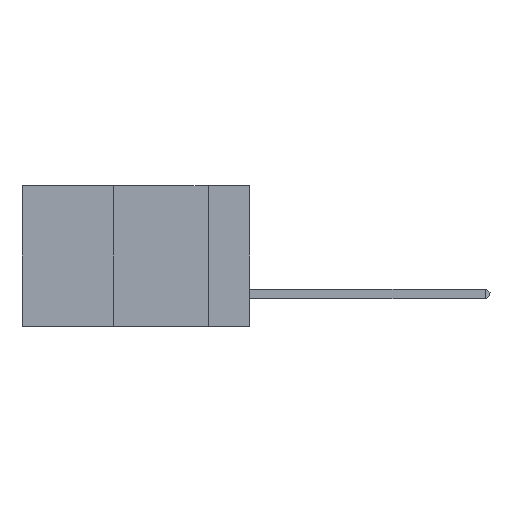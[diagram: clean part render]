
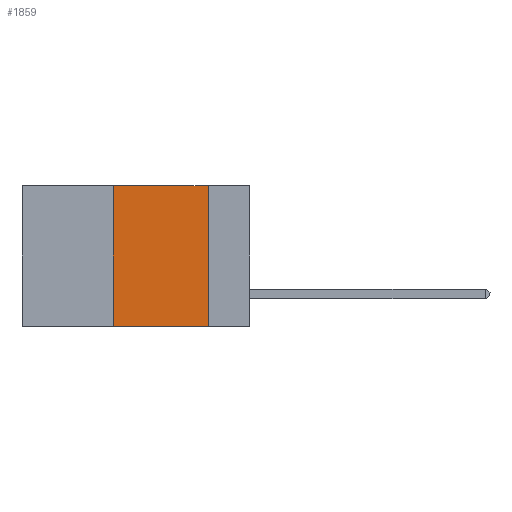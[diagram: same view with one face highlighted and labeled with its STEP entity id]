
A CAD part, left-side view. The second image highlights one B-rep face of the part: STEP entity #1859.
In plain terms, the highlighted planar face has unit normal (-1, 0, 0).
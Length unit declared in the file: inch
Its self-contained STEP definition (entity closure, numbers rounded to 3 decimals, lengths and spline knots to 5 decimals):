
#1713 = CARTESIAN_POINT ( 'NONE',  ( 0., 0.36, 0. ) ) ;
#1859 = ADVANCED_FACE ( 'NONE', ( #9444 ), #3737, .F. ) ;
#2203 = VERTEX_POINT ( 'NONE', #3024 ) ;
#2767 = DIRECTION ( 'NONE',  ( 1., 0., 0. ) ) ;
#2902 = LINE ( 'NONE', #9885, #10158 ) ;
#3024 = CARTESIAN_POINT ( 'NONE',  ( 0., 0.36, -0.37 ) ) ;
#3114 = DIRECTION ( 'NONE',  ( 0., -1., 0. ) ) ;
#3511 = EDGE_CURVE ( 'NONE', #5916, #11270, #13135, .T. ) ;
#3528 = EDGE_LOOP ( 'NONE', ( #13146, #8917, #10590, #12889 ) ) ;
#3716 = EDGE_CURVE ( 'NONE', #11270, #14510, #2902, .T. ) ;
#3737 = PLANE ( 'NONE',  #14526 ) ;
#4845 = CARTESIAN_POINT ( 'NONE',  ( 0., 0.6, 0. ) ) ;
#5087 = CARTESIAN_POINT ( 'NONE',  ( 0., 0.11, -0.37 ) ) ;
#5561 = VECTOR ( 'NONE', #5655, 39.37008 ) ;
#5655 = DIRECTION ( 'NONE',  ( 0., 0., 1. ) ) ;
#5916 = VERTEX_POINT ( 'NONE', #1713 ) ;
#6794 = LINE ( 'NONE', #11396, #5561 ) ;
#8258 = CARTESIAN_POINT ( 'NONE',  ( 0., 0.6, 0. ) ) ;
#8408 = DIRECTION ( 'NONE',  ( 0., 0., -1. ) ) ;
#8917 = ORIENTED_EDGE ( 'NONE', *, *, #3511, .F. ) ;
#8961 = CARTESIAN_POINT ( 'NONE',  ( 0., 0.11, 0. ) ) ;
#9444 = FACE_OUTER_BOUND ( 'NONE', #3528, .T. ) ;
#9885 = CARTESIAN_POINT ( 'NONE',  ( 0., 0.11, 0. ) ) ;
#10158 = VECTOR ( 'NONE', #12083, 39.37008 ) ;
#10188 = CARTESIAN_POINT ( 'NONE',  ( 0., 0.6, -0.37 ) ) ;
#10590 = ORIENTED_EDGE ( 'NONE', *, *, #12255, .F. ) ;
#11270 = VERTEX_POINT ( 'NONE', #8961 ) ;
#11348 = VECTOR ( 'NONE', #14261, 39.37008 ) ;
#11396 = CARTESIAN_POINT ( 'NONE',  ( 0., 0.36, 0. ) ) ;
#11831 = VECTOR ( 'NONE', #3114, 39.37008 ) ;
#12083 = DIRECTION ( 'NONE',  ( 0., 0., -1. ) ) ;
#12167 = EDGE_CURVE ( 'NONE', #2203, #14510, #14697, .T. ) ;
#12255 = EDGE_CURVE ( 'NONE', #2203, #5916, #6794, .T. ) ;
#12889 = ORIENTED_EDGE ( 'NONE', *, *, #12167, .T. ) ;
#13135 = LINE ( 'NONE', #4845, #11348 ) ;
#13146 = ORIENTED_EDGE ( 'NONE', *, *, #3716, .F. ) ;
#14261 = DIRECTION ( 'NONE',  ( 0., -1., 0. ) ) ;
#14510 = VERTEX_POINT ( 'NONE', #5087 ) ;
#14526 = AXIS2_PLACEMENT_3D ( 'NONE', #8258, #2767, #8408 ) ;
#14697 = LINE ( 'NONE', #10188, #11831 ) ;
